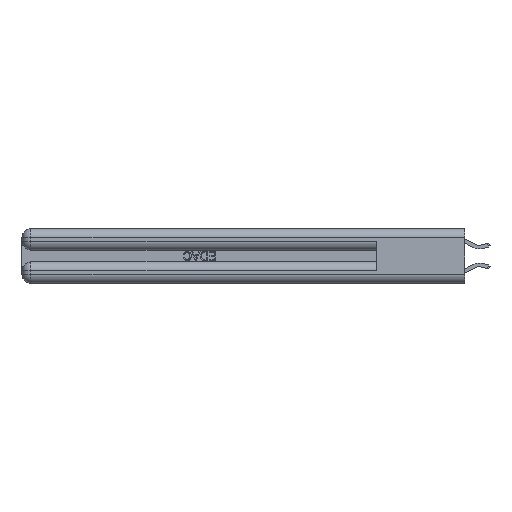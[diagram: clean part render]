
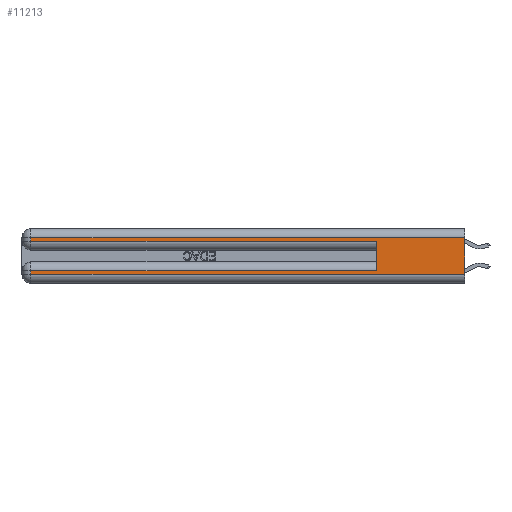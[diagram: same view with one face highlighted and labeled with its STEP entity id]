
A CAD part, left-side view. The second image highlights one B-rep face of the part: STEP entity #11213.
In plain terms, the highlighted planar face has unit normal (-1, 0, 0).
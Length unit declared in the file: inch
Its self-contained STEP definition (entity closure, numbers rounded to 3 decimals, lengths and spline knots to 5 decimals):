
#115 = LINE ( 'NONE', #27837, #8645 ) ;
#134 = EDGE_CURVE ( 'NONE', #6051, #23892, #115, .T. ) ;
#364 = CARTESIAN_POINT ( 'NONE',  ( 0., 0., 0.06 ) ) ;
#509 = CARTESIAN_POINT ( 'NONE',  ( 0., 2.94, 0.37 ) ) ;
#965 = CARTESIAN_POINT ( 'NONE',  ( 0., 2.94, 0.31 ) ) ;
#1454 = EDGE_CURVE ( 'NONE', #6051, #15145, #14415, .T. ) ;
#1758 = DIRECTION ( 'NONE',  ( 0., 1., 0. ) ) ;
#2711 = VECTOR ( 'NONE', #18008, 39.37008 ) ;
#3407 = CARTESIAN_POINT ( 'NONE',  ( 0., 2.94, 0.085 ) ) ;
#4718 = PLANE ( 'NONE',  #10335 ) ;
#5086 = CARTESIAN_POINT ( 'NONE',  ( 0., 2.94, 0.06 ) ) ;
#6051 = VERTEX_POINT ( 'NONE', #34536 ) ;
#6097 = ORIENTED_EDGE ( 'NONE', *, *, #9923, .T. ) ;
#6605 = DIRECTION ( 'NONE',  ( 0., -1., 0. ) ) ;
#7793 = ORIENTED_EDGE ( 'NONE', *, *, #19222, .T. ) ;
#8244 = ORIENTED_EDGE ( 'NONE', *, *, #33855, .T. ) ;
#8606 = LINE ( 'NONE', #28278, #21920 ) ;
#8645 = VECTOR ( 'NONE', #25153, 39.37008 ) ;
#8953 = CARTESIAN_POINT ( 'NONE',  ( 0., 0., 0.06 ) ) ;
#8982 = VERTEX_POINT ( 'NONE', #26935 ) ;
#9142 = DIRECTION ( 'NONE',  ( 0., 0., -1. ) ) ;
#9478 = LINE ( 'NONE', #25107, #33763 ) ;
#9923 = EDGE_CURVE ( 'NONE', #25278, #21101, #8606, .T. ) ;
#10335 = AXIS2_PLACEMENT_3D ( 'NONE', #21339, #24027, #13271 ) ;
#10764 = FACE_OUTER_BOUND ( 'NONE', #25307, .T. ) ;
#11213 = ADVANCED_FACE ( 'NONE', ( #10764 ), #4718, .F. ) ;
#11418 = DIRECTION ( 'NONE',  ( 0., 0., -1. ) ) ;
#11518 = VECTOR ( 'NONE', #27845, 39.37008 ) ;
#11966 = LINE ( 'NONE', #8953, #12134 ) ;
#12134 = VECTOR ( 'NONE', #6605, 39.37008 ) ;
#13271 = DIRECTION ( 'NONE',  ( 0., 0., -1. ) ) ;
#13850 = EDGE_CURVE ( 'NONE', #14687, #8982, #15323, .T. ) ;
#14021 = ORIENTED_EDGE ( 'NONE', *, *, #13850, .T. ) ;
#14415 = LINE ( 'NONE', #24793, #11518 ) ;
#14687 = VERTEX_POINT ( 'NONE', #34542 ) ;
#15078 = ORIENTED_EDGE ( 'NONE', *, *, #1454, .T. ) ;
#15145 = VERTEX_POINT ( 'NONE', #965 ) ;
#15317 = VECTOR ( 'NONE', #1758, 39.37008 ) ;
#15323 = LINE ( 'NONE', #31785, #2711 ) ;
#16513 = DIRECTION ( 'NONE',  ( 0., 0., 1. ) ) ;
#16604 = EDGE_CURVE ( 'NONE', #32483, #25278, #18032, .T. ) ;
#16960 = ORIENTED_EDGE ( 'NONE', *, *, #134, .F. ) ;
#18008 = DIRECTION ( 'NONE',  ( 0., -1., 0. ) ) ;
#18032 = LINE ( 'NONE', #26263, #15317 ) ;
#19222 = EDGE_CURVE ( 'NONE', #15145, #14687, #27708, .T. ) ;
#21101 = VERTEX_POINT ( 'NONE', #5086 ) ;
#21339 = CARTESIAN_POINT ( 'NONE',  ( 0., 0., 0.37 ) ) ;
#21920 = VECTOR ( 'NONE', #9142, 39.37008 ) ;
#23396 = ORIENTED_EDGE ( 'NONE', *, *, #30089, .F. ) ;
#23892 = VERTEX_POINT ( 'NONE', #364 ) ;
#24027 = DIRECTION ( 'NONE',  ( 1., 0., 0. ) ) ;
#24793 = CARTESIAN_POINT ( 'NONE',  ( 0., 0., 0.31 ) ) ;
#24922 = ORIENTED_EDGE ( 'NONE', *, *, #16604, .T. ) ;
#25107 = CARTESIAN_POINT ( 'NONE',  ( 0., 0.6, 0.145 ) ) ;
#25153 = DIRECTION ( 'NONE',  ( 0., 0., -1. ) ) ;
#25179 = VECTOR ( 'NONE', #11418, 39.37008 ) ;
#25278 = VERTEX_POINT ( 'NONE', #3407 ) ;
#25307 = EDGE_LOOP ( 'NONE', ( #16960, #15078, #7793, #14021, #23396, #24922, #6097, #8244 ) ) ;
#26263 = CARTESIAN_POINT ( 'NONE',  ( 0., 0., 0.085 ) ) ;
#26935 = CARTESIAN_POINT ( 'NONE',  ( 0., 0.6, 0.285 ) ) ;
#27708 = LINE ( 'NONE', #509, #25179 ) ;
#27837 = CARTESIAN_POINT ( 'NONE',  ( 0., 0., 0.37 ) ) ;
#27845 = DIRECTION ( 'NONE',  ( 0., 1., 0. ) ) ;
#28278 = CARTESIAN_POINT ( 'NONE',  ( 0., 2.94, 0.37 ) ) ;
#30089 = EDGE_CURVE ( 'NONE', #32483, #8982, #9478, .T. ) ;
#31785 = CARTESIAN_POINT ( 'NONE',  ( 0., 0., 0.285 ) ) ;
#32483 = VERTEX_POINT ( 'NONE', #33467 ) ;
#33467 = CARTESIAN_POINT ( 'NONE',  ( 0., 0.6, 0.085 ) ) ;
#33763 = VECTOR ( 'NONE', #16513, 39.37008 ) ;
#33855 = EDGE_CURVE ( 'NONE', #21101, #23892, #11966, .T. ) ;
#34536 = CARTESIAN_POINT ( 'NONE',  ( 0., 0., 0.31 ) ) ;
#34542 = CARTESIAN_POINT ( 'NONE',  ( 0., 2.94, 0.285 ) ) ;
